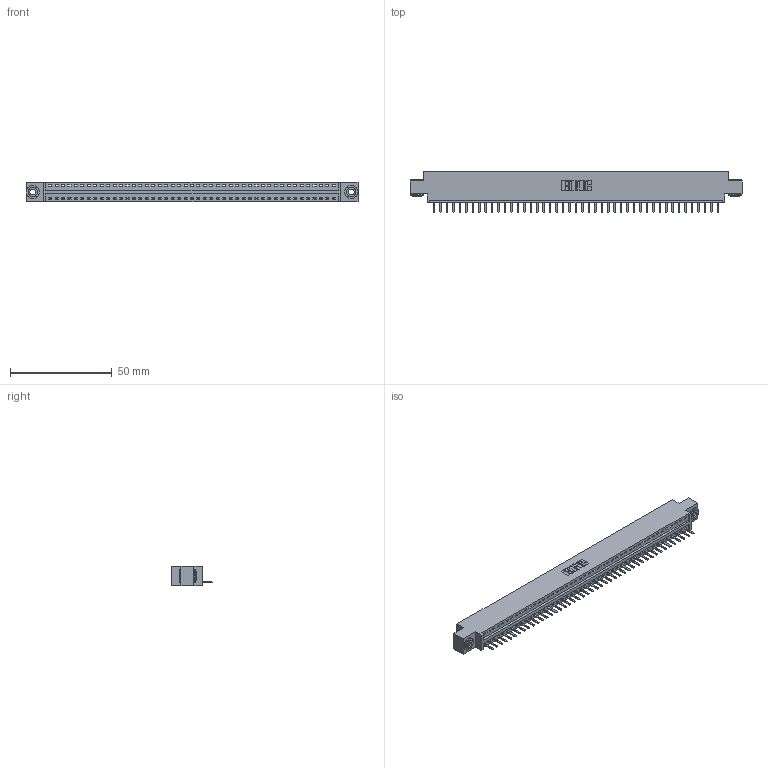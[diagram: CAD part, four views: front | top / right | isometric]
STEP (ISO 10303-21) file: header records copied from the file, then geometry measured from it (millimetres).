
FILE_DESCRIPTION (( 'STEP AP203' ), '1' );
FILE_NAME ('396-045-520-603.STEP', '2019-10-28T00:15:42', ( '' ), ( '' ), 'SwSTEP 2.0', 'SolidWorks 2016', '' );
FILE_SCHEMA (( 'CONFIG_CONTROL_DESIGN' ));
Length unit declared in the file: inch
Products named in the file (4): 345-292-001_345-293-120; 345-250-002_345-250-002-102; 396-045-520-603; 346 Part_0.170 Offset - 0.156 Dia-TH
Assembly tree (48 placements, depth 2):
  396-045-520-603
    346 Part_0.170 Offset - 0.156 Dia-TH
    345-292-001_345-293-120  x45
    345-250-002_345-250-002-102  x2
Bounding box: 163.45 x 20.02 x 9.4 mm (x, y, z)
Volume: 15401.7 mm3; surface area: 19229.9 mm2
Topology: 48 solids, 48 shells, 2954 faces, 8697 edges, 5674 vertices
Faces by surface type: plane 1980, cylinder 966, cone 8
Entity records: 28420 total; most frequent: CARTESIAN_POINT 4862, ORIENTED_EDGE 4822, DIRECTION 4303, EDGE_CURVE 2411, VECTOR 2071, LINE 2071, VERTEX_POINT 1602, AXIS2_PLACEMENT_3D 1116
